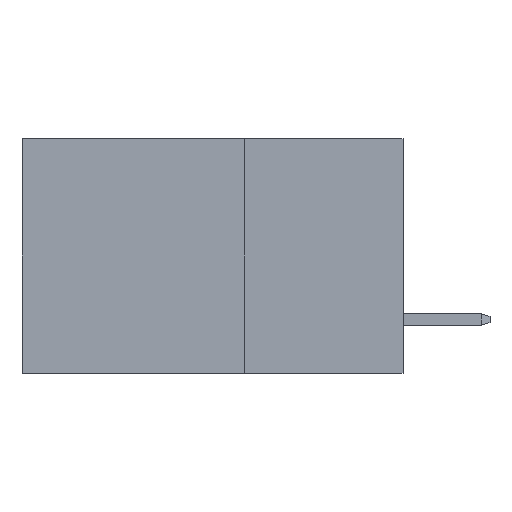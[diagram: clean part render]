
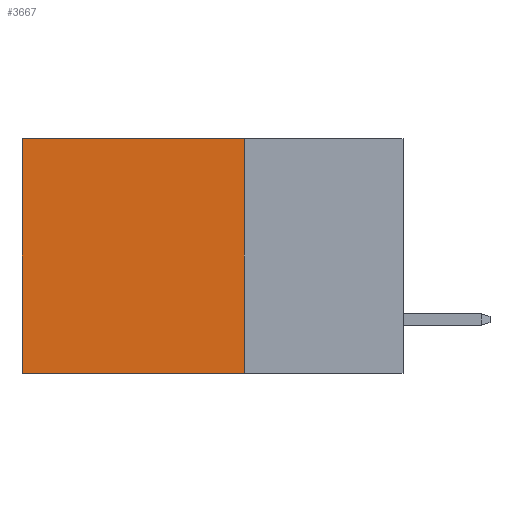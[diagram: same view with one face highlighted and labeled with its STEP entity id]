
A CAD part, left-side view. The second image highlights one B-rep face of the part: STEP entity #3667.
In plain terms, the highlighted planar face has unit normal (-1, 0, 0).
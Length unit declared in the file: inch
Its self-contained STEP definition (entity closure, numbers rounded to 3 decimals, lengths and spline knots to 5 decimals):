
#24 = VERTEX_POINT ( 'NONE', #3062 ) ;
#42 = CARTESIAN_POINT ( 'NONE',  ( 0.2875, 0.25, 0. ) ) ;
#361 = DIRECTION ( 'NONE',  ( 1., 0., 0. ) ) ;
#511 = CARTESIAN_POINT ( 'NONE',  ( 0.2875, 0.25, -0.37 ) ) ;
#1879 = DIRECTION ( 'NONE',  ( 0., 1., 0. ) ) ;
#2204 = VECTOR ( 'NONE', #6108, 39.37008 ) ;
#2605 = AXIS2_PLACEMENT_3D ( 'NONE', #9978, #361, #5963 ) ;
#2800 = CARTESIAN_POINT ( 'NONE',  ( 0.2875, 0.6, -0.37 ) ) ;
#3062 = CARTESIAN_POINT ( 'NONE',  ( 0.2875, 0.6, 0. ) ) ;
#3168 = EDGE_LOOP ( 'NONE', ( #12793, #6271, #14324, #5919 ) ) ;
#3626 = LINE ( 'NONE', #12003, #17510 ) ;
#3667 = ADVANCED_FACE ( 'NONE', ( #4302 ), #16971, .F. ) ;
#4302 = FACE_OUTER_BOUND ( 'NONE', #3168, .T. ) ;
#5317 = VECTOR ( 'NONE', #13498, 39.37008 ) ;
#5588 = EDGE_CURVE ( 'NONE', #24, #16887, #3626, .T. ) ;
#5919 = ORIENTED_EDGE ( 'NONE', *, *, #17011, .T. ) ;
#5963 = DIRECTION ( 'NONE',  ( 0., 0., -1. ) ) ;
#6108 = DIRECTION ( 'NONE',  ( 0., 1., 0. ) ) ;
#6271 = ORIENTED_EDGE ( 'NONE', *, *, #10045, .F. ) ;
#6397 = EDGE_CURVE ( 'NONE', #8780, #9691, #9252, .T. ) ;
#8780 = VERTEX_POINT ( 'NONE', #42 ) ;
#9252 = LINE ( 'NONE', #10621, #5317 ) ;
#9691 = VERTEX_POINT ( 'NONE', #511 ) ;
#9978 = CARTESIAN_POINT ( 'NONE',  ( 0.2875, 0.25, 0. ) ) ;
#10045 = EDGE_CURVE ( 'NONE', #9691, #16887, #16087, .T. ) ;
#10621 = CARTESIAN_POINT ( 'NONE',  ( 0.2875, 0.25, 0. ) ) ;
#12003 = CARTESIAN_POINT ( 'NONE',  ( 0.2875, 0.6, 0. ) ) ;
#12793 = ORIENTED_EDGE ( 'NONE', *, *, #5588, .T. ) ;
#13003 = CARTESIAN_POINT ( 'NONE',  ( 0.2875, 0.25, -0.37 ) ) ;
#13498 = DIRECTION ( 'NONE',  ( 0., 0., -1. ) ) ;
#14290 = CARTESIAN_POINT ( 'NONE',  ( 0.2875, 0.25, 0. ) ) ;
#14324 = ORIENTED_EDGE ( 'NONE', *, *, #6397, .F. ) ;
#15644 = LINE ( 'NONE', #14290, #17405 ) ;
#16087 = LINE ( 'NONE', #13003, #2204 ) ;
#16887 = VERTEX_POINT ( 'NONE', #2800 ) ;
#16971 = PLANE ( 'NONE',  #2605 ) ;
#17011 = EDGE_CURVE ( 'NONE', #8780, #24, #15644, .T. ) ;
#17405 = VECTOR ( 'NONE', #1879, 39.37008 ) ;
#17510 = VECTOR ( 'NONE', #17761, 39.37008 ) ;
#17761 = DIRECTION ( 'NONE',  ( 0., 0., -1. ) ) ;
